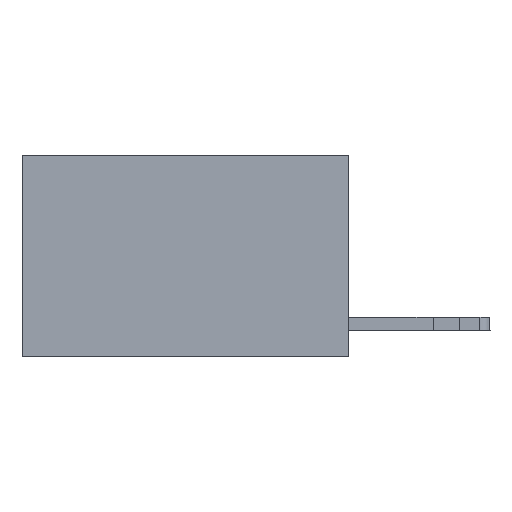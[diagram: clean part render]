
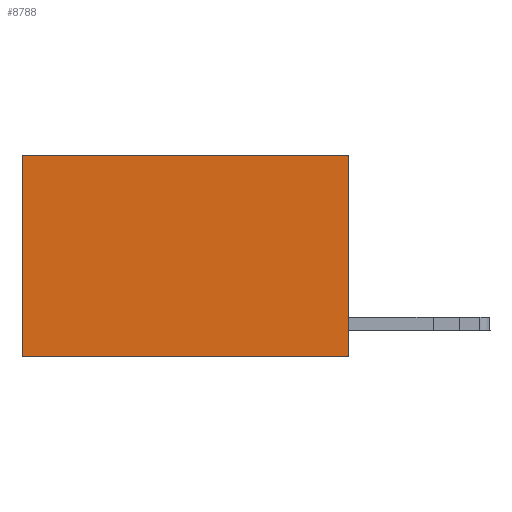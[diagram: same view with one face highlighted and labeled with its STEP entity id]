
A CAD part, left-side view. The second image highlights one B-rep face of the part: STEP entity #8788.
In plain terms, the highlighted planar face has unit normal (-1, 0, 0).
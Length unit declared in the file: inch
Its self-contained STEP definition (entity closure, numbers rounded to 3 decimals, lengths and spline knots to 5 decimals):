
#1233 = VECTOR ( 'NONE', #5234, 39.37008 ) ;
#1500 = ORIENTED_EDGE ( 'NONE', *, *, #4510, .T. ) ;
#1719 = CARTESIAN_POINT ( 'NONE',  ( 0.2625, 0.6, 0. ) ) ;
#1814 = ORIENTED_EDGE ( 'NONE', *, *, #3659, .T. ) ;
#2009 = CARTESIAN_POINT ( 'NONE',  ( 0.2625, 0.6, -0.37 ) ) ;
#2606 = LINE ( 'NONE', #9504, #7834 ) ;
#3650 = FACE_OUTER_BOUND ( 'NONE', #10355, .T. ) ;
#3659 = EDGE_CURVE ( 'NONE', #7604, #4472, #9616, .T. ) ;
#4164 = CARTESIAN_POINT ( 'NONE',  ( 0.2625, 0.6, 0. ) ) ;
#4315 = VECTOR ( 'NONE', #7591, 39.37008 ) ;
#4393 = ORIENTED_EDGE ( 'NONE', *, *, #9712, .F. ) ;
#4472 = VERTEX_POINT ( 'NONE', #1719 ) ;
#4510 = EDGE_CURVE ( 'NONE', #4472, #6750, #6932, .T. ) ;
#5234 = DIRECTION ( 'NONE',  ( 0., 0., -1. ) ) ;
#5321 = VECTOR ( 'NONE', #11297, 39.37008 ) ;
#5440 = CARTESIAN_POINT ( 'NONE',  ( 0.2625, 0., 0. ) ) ;
#6750 = VERTEX_POINT ( 'NONE', #2009 ) ;
#6932 = LINE ( 'NONE', #4164, #1233 ) ;
#7454 = CARTESIAN_POINT ( 'NONE',  ( 0.2625, 0., -0.37 ) ) ;
#7591 = DIRECTION ( 'NONE',  ( 0., 1., 0. ) ) ;
#7604 = VERTEX_POINT ( 'NONE', #9200 ) ;
#7644 = DIRECTION ( 'NONE',  ( 0., 1., 0. ) ) ;
#7656 = DIRECTION ( 'NONE',  ( 1., 0., 0. ) ) ;
#7834 = VECTOR ( 'NONE', #7644, 39.37008 ) ;
#8496 = VERTEX_POINT ( 'NONE', #7454 ) ;
#8515 = EDGE_CURVE ( 'NONE', #7604, #8496, #12479, .T. ) ;
#8788 = ADVANCED_FACE ( 'NONE', ( #3650 ), #9553, .F. ) ;
#9200 = CARTESIAN_POINT ( 'NONE',  ( 0.2625, 0., 0. ) ) ;
#9504 = CARTESIAN_POINT ( 'NONE',  ( 0.2625, 0., -0.37 ) ) ;
#9553 = PLANE ( 'NONE',  #10450 ) ;
#9616 = LINE ( 'NONE', #12438, #4315 ) ;
#9712 = EDGE_CURVE ( 'NONE', #8496, #6750, #2606, .T. ) ;
#10355 = EDGE_LOOP ( 'NONE', ( #1500, #4393, #12250, #1814 ) ) ;
#10450 = AXIS2_PLACEMENT_3D ( 'NONE', #10526, #7656, #11503 ) ;
#10526 = CARTESIAN_POINT ( 'NONE',  ( 0.2625, 0., 0. ) ) ;
#11297 = DIRECTION ( 'NONE',  ( 0., 0., -1. ) ) ;
#11503 = DIRECTION ( 'NONE',  ( 0., 0., -1. ) ) ;
#12250 = ORIENTED_EDGE ( 'NONE', *, *, #8515, .F. ) ;
#12438 = CARTESIAN_POINT ( 'NONE',  ( 0.2625, 0., 0. ) ) ;
#12479 = LINE ( 'NONE', #5440, #5321 ) ;
